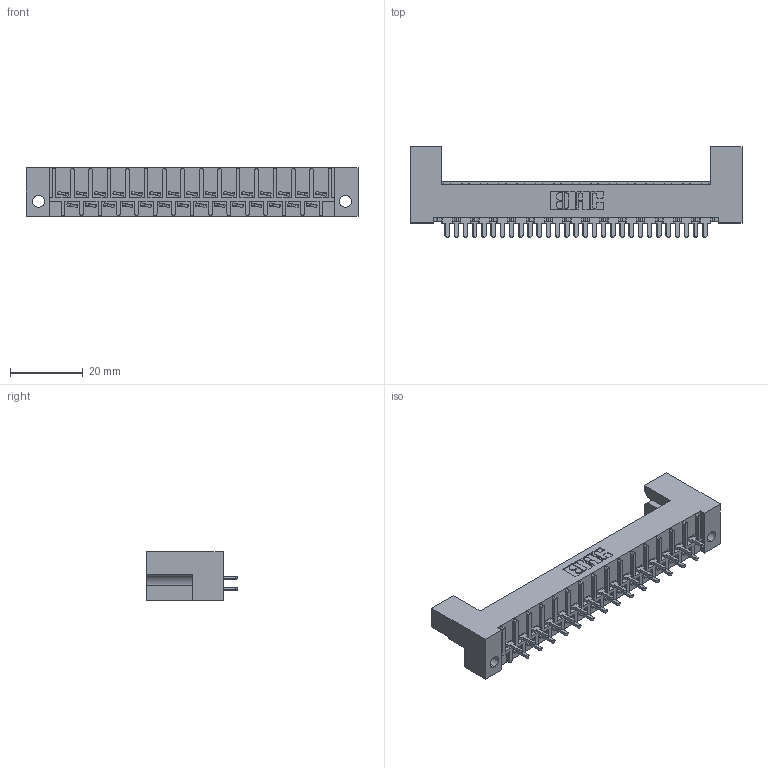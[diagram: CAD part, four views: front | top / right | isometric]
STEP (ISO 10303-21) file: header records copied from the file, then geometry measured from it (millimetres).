
FILE_DESCRIPTION (( 'STEP AP203' ), '1' );
FILE_NAME ('408-029-521-222.STEP', '2019-11-04T18:58:46', ( '' ), ( '' ), 'SwSTEP 2.0', 'SolidWorks 2016', '' );
FILE_SCHEMA (( 'CONFIG_CONTROL_DESIGN' ));
Length unit declared in the file: inch
Products named in the file (3): 408-290-001_408-290-121; 408-029-521-222; 408 Part_029 - 2
Assembly tree (30 placements, depth 2):
  408-029-521-222
    408 Part_029 - 2
    408-290-001_408-290-121  x29
Bounding box: 91.59 x 24.94 x 13.49 mm (x, y, z)
Volume: 11635.8 mm3; surface area: 13181.2 mm2
Topology: 30 solids, 30 shells, 1737 faces, 4777 edges, 3106 vertices
Faces by surface type: plane 1307, cylinder 314, bspline 116
Entity records: 23470 total; most frequent: CARTESIAN_POINT 4053, ORIENTED_EDGE 3954, DIRECTION 3609, EDGE_CURVE 1977, VECTOR 1741, LINE 1741, VERTEX_POINT 1314, AXIS2_PLACEMENT_3D 934
